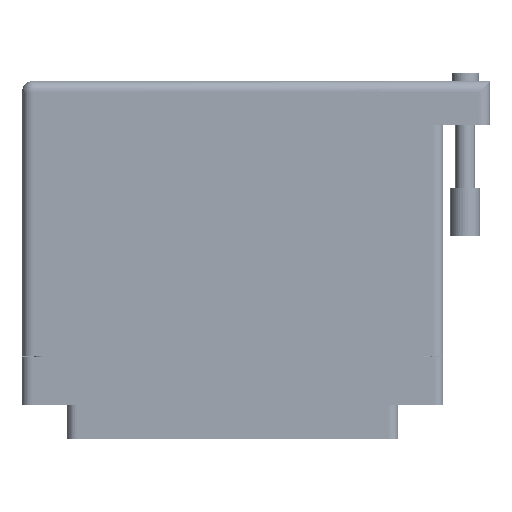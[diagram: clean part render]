
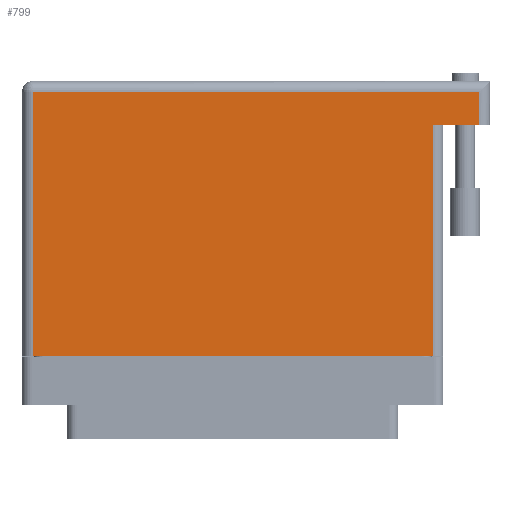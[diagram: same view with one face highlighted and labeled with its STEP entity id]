
A CAD part, front view. The second image highlights one B-rep face of the part: STEP entity #799.
In plain terms, the highlighted face is planar.
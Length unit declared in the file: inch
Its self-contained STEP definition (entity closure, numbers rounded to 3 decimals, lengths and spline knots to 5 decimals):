
#216 = AXIS2_PLACEMENT_3D ( 'NONE', #32713, #43557, #38395 ) ;
#799 = ADVANCED_FACE ( 'NONE', ( #68770 ), #54924, .F. ) ;
#3588 = ORIENTED_EDGE ( 'NONE', *, *, #47859, .F. ) ;
#4184 = LINE ( 'NONE', #67841, #47415 ) ;
#6696 = DIRECTION ( 'NONE',  ( 0., 1., 0. ) ) ;
#8745 = ORIENTED_EDGE ( 'NONE', *, *, #68322, .T. ) ;
#10058 = LINE ( 'NONE', #65699, #54072 ) ;
#11145 = EDGE_CURVE ( 'NONE', #21706, #36156, #4184, .T. ) ;
#15907 = LINE ( 'NONE', #16752, #47954 ) ;
#16752 = CARTESIAN_POINT ( 'NONE',  ( 1.289, 1.395, 0.617 ) ) ;
#18011 = DIRECTION ( 'NONE',  ( 0., -1., 0. ) ) ;
#21706 = VERTEX_POINT ( 'NONE', #22076 ) ;
#21943 = CARTESIAN_POINT ( 'NONE',  ( -1.289, 1.605, 0.617 ) ) ;
#22076 = CARTESIAN_POINT ( 'NONE',  ( -1.289, -0.1, 0.617 ) ) ;
#24414 = CARTESIAN_POINT ( 'NONE',  ( 1.589, 1.675, 0.617 ) ) ;
#25105 = DIRECTION ( 'NONE',  ( 0., 1., 0. ) ) ;
#26319 = LINE ( 'NONE', #31884, #64297 ) ;
#27037 = EDGE_CURVE ( 'NONE', #69172, #21706, #39406, .T. ) ;
#29502 = CARTESIAN_POINT ( 'NONE',  ( 1.589, 1.395, 0.617 ) ) ;
#30108 = VERTEX_POINT ( 'NONE', #36454 ) ;
#30867 = VERTEX_POINT ( 'NONE', #63515 ) ;
#31884 = CARTESIAN_POINT ( 'NONE',  ( 1.659, 1.395, 0.617 ) ) ;
#32713 = CARTESIAN_POINT ( 'NONE',  ( -1.359, 1.675, 0.617 ) ) ;
#34643 = ORIENTED_EDGE ( 'NONE', *, *, #60320, .T. ) ;
#36156 = VERTEX_POINT ( 'NONE', #47138 ) ;
#36454 = CARTESIAN_POINT ( 'NONE',  ( 1.289, 1.395, 0.617 ) ) ;
#38395 = DIRECTION ( 'NONE',  ( -1., 0., 0. ) ) ;
#39406 = LINE ( 'NONE', #60060, #52151 ) ;
#41913 = LINE ( 'NONE', #24414, #44373 ) ;
#42409 = ORIENTED_EDGE ( 'NONE', *, *, #27037, .T. ) ;
#42720 = ORIENTED_EDGE ( 'NONE', *, *, #11145, .T. ) ;
#43557 = DIRECTION ( 'NONE',  ( 0., 0., -1. ) ) ;
#44373 = VECTOR ( 'NONE', #25105, 39.37008 ) ;
#45042 = EDGE_CURVE ( 'NONE', #30867, #69172, #10058, .T. ) ;
#47138 = CARTESIAN_POINT ( 'NONE',  ( 1.289, -0.1, 0.617 ) ) ;
#47415 = VECTOR ( 'NONE', #61944, 39.37008 ) ;
#47859 = EDGE_CURVE ( 'NONE', #56459, #30108, #26319, .T. ) ;
#47954 = VECTOR ( 'NONE', #6696, 39.37008 ) ;
#52151 = VECTOR ( 'NONE', #18011, 39.37008 ) ;
#53179 = DIRECTION ( 'NONE',  ( -1., 0., 0. ) ) ;
#54072 = VECTOR ( 'NONE', #65452, 39.37008 ) ;
#54924 = PLANE ( 'NONE',  #216 ) ;
#55620 = EDGE_LOOP ( 'NONE', ( #42720, #8745, #3588, #34643, #62098, #42409 ) ) ;
#56459 = VERTEX_POINT ( 'NONE', #29502 ) ;
#60060 = CARTESIAN_POINT ( 'NONE',  ( -1.289, -0.1, 0.617 ) ) ;
#60320 = EDGE_CURVE ( 'NONE', #56459, #30867, #41913, .T. ) ;
#61944 = DIRECTION ( 'NONE',  ( 1., 0., 0. ) ) ;
#62098 = ORIENTED_EDGE ( 'NONE', *, *, #45042, .T. ) ;
#63515 = CARTESIAN_POINT ( 'NONE',  ( 1.589, 1.605, 0.617 ) ) ;
#64297 = VECTOR ( 'NONE', #53179, 39.37008 ) ;
#65452 = DIRECTION ( 'NONE',  ( -1., 0., 0. ) ) ;
#65699 = CARTESIAN_POINT ( 'NONE',  ( -1.359, 1.605, 0.617 ) ) ;
#67841 = CARTESIAN_POINT ( 'NONE',  ( -1.359, -0.1, 0.617 ) ) ;
#68322 = EDGE_CURVE ( 'NONE', #36156, #30108, #15907, .T. ) ;
#68770 = FACE_OUTER_BOUND ( 'NONE', #55620, .T. ) ;
#69172 = VERTEX_POINT ( 'NONE', #21943 ) ;
